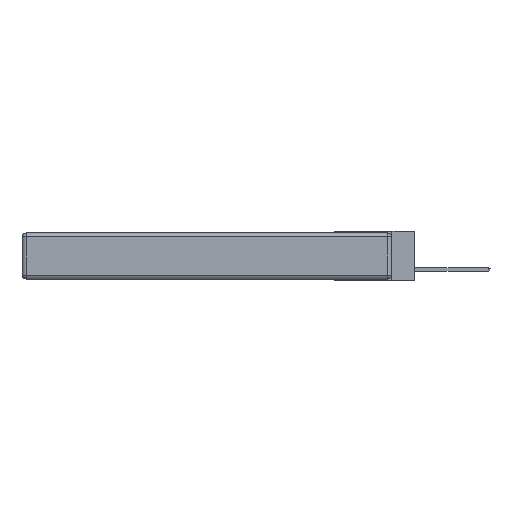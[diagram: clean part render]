
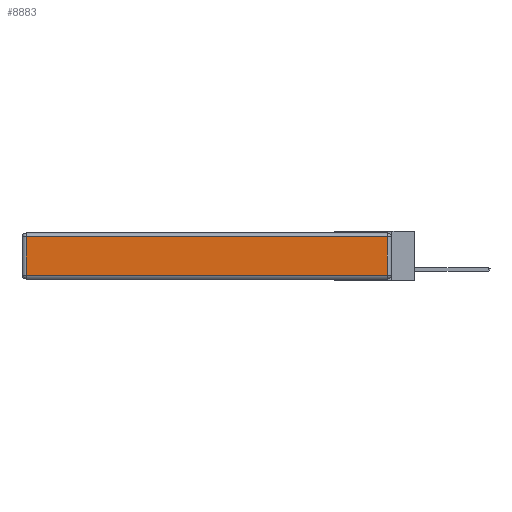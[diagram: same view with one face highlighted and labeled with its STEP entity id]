
A CAD part, left-side view. The second image highlights one B-rep face of the part: STEP entity #8883.
In plain terms, the highlighted planar face has unit normal (-1, 0, 0).
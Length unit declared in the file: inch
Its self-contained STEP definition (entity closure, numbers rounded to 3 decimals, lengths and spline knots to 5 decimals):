
#184 = ORIENTED_EDGE ( 'NONE', *, *, #2175, .T. ) ;
#990 = CARTESIAN_POINT ( 'NONE',  ( 0., 0.03, -0.343 ) ) ;
#1589 = VERTEX_POINT ( 'NONE', #13547 ) ;
#2175 = EDGE_CURVE ( 'NONE', #17664, #1589, #3776, .T. ) ;
#2496 = LINE ( 'NONE', #19412, #17020 ) ;
#3059 = LINE ( 'NONE', #3408, #10338 ) ;
#3391 = DIRECTION ( 'NONE',  ( 0., 1., 0. ) ) ;
#3408 = CARTESIAN_POINT ( 'NONE',  ( 0., 2.72, -0.343 ) ) ;
#3448 = AXIS2_PLACEMENT_3D ( 'NONE', #19300, #4407, #5722 ) ;
#3776 = LINE ( 'NONE', #990, #16481 ) ;
#4407 = DIRECTION ( 'NONE',  ( -1., 0., 0. ) ) ;
#5136 = FACE_OUTER_BOUND ( 'NONE', #17235, .T. ) ;
#5431 = DIRECTION ( 'NONE',  ( 0., 0., 1. ) ) ;
#5722 = DIRECTION ( 'NONE',  ( 0., 0., 1. ) ) ;
#6500 = CARTESIAN_POINT ( 'NONE',  ( 0., 0.03, -0.313 ) ) ;
#6668 = VERTEX_POINT ( 'NONE', #13997 ) ;
#7419 = ORIENTED_EDGE ( 'NONE', *, *, #14960, .T. ) ;
#7752 = LINE ( 'NONE', #10817, #18758 ) ;
#8808 = PLANE ( 'NONE',  #3448 ) ;
#8883 = ADVANCED_FACE ( 'NONE', ( #5136 ), #8808, .T. ) ;
#9740 = VERTEX_POINT ( 'NONE', #16081 ) ;
#10338 = VECTOR ( 'NONE', #13914, 39.37008 ) ;
#10817 = CARTESIAN_POINT ( 'NONE',  ( 0., 2.75, -0.03 ) ) ;
#12253 = EDGE_CURVE ( 'NONE', #6668, #17664, #2496, .T. ) ;
#13547 = CARTESIAN_POINT ( 'NONE',  ( 0., 0.03, -0.03 ) ) ;
#13914 = DIRECTION ( 'NONE',  ( 0., 0., -1. ) ) ;
#13997 = CARTESIAN_POINT ( 'NONE',  ( 0., 2.72, -0.313 ) ) ;
#14960 = EDGE_CURVE ( 'NONE', #9740, #6668, #3059, .T. ) ;
#15504 = ORIENTED_EDGE ( 'NONE', *, *, #16158, .T. ) ;
#16081 = CARTESIAN_POINT ( 'NONE',  ( 0., 2.72, -0.03 ) ) ;
#16158 = EDGE_CURVE ( 'NONE', #1589, #9740, #7752, .T. ) ;
#16324 = DIRECTION ( 'NONE',  ( 0., -1., 0. ) ) ;
#16481 = VECTOR ( 'NONE', #5431, 39.37008 ) ;
#17020 = VECTOR ( 'NONE', #16324, 39.37008 ) ;
#17028 = ORIENTED_EDGE ( 'NONE', *, *, #12253, .T. ) ;
#17235 = EDGE_LOOP ( 'NONE', ( #17028, #184, #15504, #7419 ) ) ;
#17664 = VERTEX_POINT ( 'NONE', #6500 ) ;
#18758 = VECTOR ( 'NONE', #3391, 39.37008 ) ;
#19300 = CARTESIAN_POINT ( 'NONE',  ( 0., 0., -0.343 ) ) ;
#19412 = CARTESIAN_POINT ( 'NONE',  ( 0., 0., -0.313 ) ) ;
